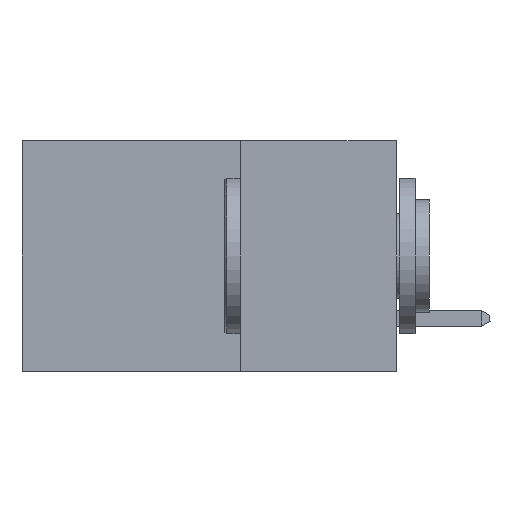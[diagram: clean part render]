
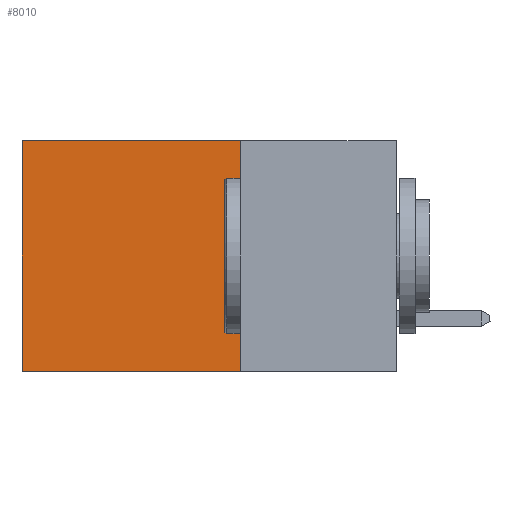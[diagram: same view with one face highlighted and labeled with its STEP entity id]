
A CAD part, left-side view. The second image highlights one B-rep face of the part: STEP entity #8010.
In plain terms, the highlighted planar face has unit normal (-1, 0, 0).
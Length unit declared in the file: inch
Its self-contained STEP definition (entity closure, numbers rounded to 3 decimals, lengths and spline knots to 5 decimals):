
#11 = DIRECTION ( 'NONE',  ( 0., 0., -1. ) ) ;
#82 = CARTESIAN_POINT ( 'NONE',  ( 0.298, 0.25, 0. ) ) ;
#105 = CARTESIAN_POINT ( 'NONE',  ( 0.298, 0.25, -0.37 ) ) ;
#1968 = CARTESIAN_POINT ( 'NONE',  ( 0.298, 0.6, 0. ) ) ;
#2689 = ORIENTED_EDGE ( 'NONE', *, *, #10836, .T. ) ;
#2807 = AXIS2_PLACEMENT_3D ( 'NONE', #11896, #14195, #11 ) ;
#3208 = ORIENTED_EDGE ( 'NONE', *, *, #5172, .T. ) ;
#3561 = DIRECTION ( 'NONE',  ( 0., 1., 0. ) ) ;
#4274 = LINE ( 'NONE', #12904, #9797 ) ;
#5172 = EDGE_CURVE ( 'NONE', #17700, #12400, #10494, .T. ) ;
#5437 = DIRECTION ( 'NONE',  ( 0., 1., 0. ) ) ;
#6139 = VERTEX_POINT ( 'NONE', #105 ) ;
#6143 = CARTESIAN_POINT ( 'NONE',  ( 0.298, 0.25, 0. ) ) ;
#6602 = EDGE_LOOP ( 'NONE', ( #2689, #14145, #9709, #3208 ) ) ;
#8010 = ADVANCED_FACE ( 'NONE', ( #11728 ), #25640, .F. ) ;
#8071 = CARTESIAN_POINT ( 'NONE',  ( 0.298, 0.6, -0.37 ) ) ;
#8667 = VECTOR ( 'NONE', #29437, 39.37008 ) ;
#9709 = ORIENTED_EDGE ( 'NONE', *, *, #30065, .F. ) ;
#9797 = VECTOR ( 'NONE', #3561, 39.37008 ) ;
#10494 = LINE ( 'NONE', #82, #21995 ) ;
#10836 = EDGE_CURVE ( 'NONE', #12400, #20405, #29091, .T. ) ;
#11402 = DIRECTION ( 'NONE',  ( 0., 0., -1. ) ) ;
#11728 = FACE_OUTER_BOUND ( 'NONE', #6602, .T. ) ;
#11896 = CARTESIAN_POINT ( 'NONE',  ( 0.298, 0.25, 0. ) ) ;
#12400 = VERTEX_POINT ( 'NONE', #28987 ) ;
#12904 = CARTESIAN_POINT ( 'NONE',  ( 0.298, 0.25, -0.37 ) ) ;
#14145 = ORIENTED_EDGE ( 'NONE', *, *, #28146, .F. ) ;
#14195 = DIRECTION ( 'NONE',  ( 1., 0., 0. ) ) ;
#17700 = VERTEX_POINT ( 'NONE', #6143 ) ;
#20405 = VERTEX_POINT ( 'NONE', #8071 ) ;
#21995 = VECTOR ( 'NONE', #5437, 39.37008 ) ;
#23064 = VECTOR ( 'NONE', #11402, 39.37008 ) ;
#25640 = PLANE ( 'NONE',  #2807 ) ;
#27010 = LINE ( 'NONE', #27210, #8667 ) ;
#27210 = CARTESIAN_POINT ( 'NONE',  ( 0.298, 0.25, 0. ) ) ;
#28146 = EDGE_CURVE ( 'NONE', #6139, #20405, #4274, .T. ) ;
#28987 = CARTESIAN_POINT ( 'NONE',  ( 0.298, 0.6, 0. ) ) ;
#29091 = LINE ( 'NONE', #1968, #23064 ) ;
#29437 = DIRECTION ( 'NONE',  ( 0., 0., -1. ) ) ;
#30065 = EDGE_CURVE ( 'NONE', #17700, #6139, #27010, .T. ) ;
